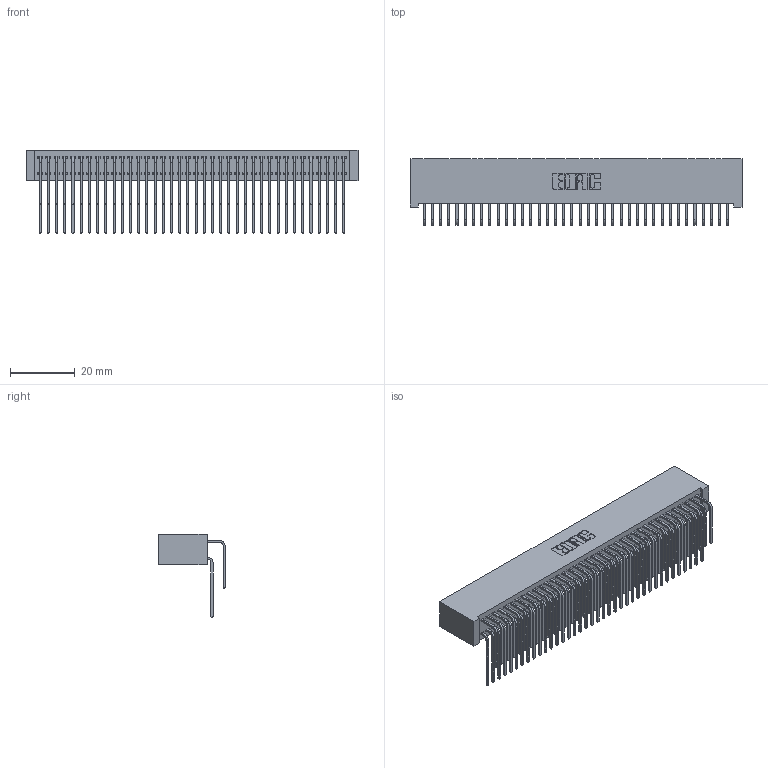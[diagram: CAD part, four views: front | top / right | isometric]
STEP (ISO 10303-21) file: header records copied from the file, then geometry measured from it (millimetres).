
FILE_DESCRIPTION (( 'STEP AP203' ), '1' );
FILE_NAME ('392-076-559-201.STEP', '2018-08-18T01:47:36', ( '' ), ( '' ), 'SwSTEP 2.0', 'SolidWorks 2016', '' );
FILE_SCHEMA (( 'CONFIG_CONTROL_DESIGN' ));
Length unit declared in the file: inch
Products named in the file (4): 342 Part_Lugless; 345-292-001_558 559 Tail - 1; 345-292-001_559 Tail - 2; 392-076-559-201
Assembly tree (77 placements, depth 2):
  392-076-559-201
    342 Part_Lugless
    345-292-001_558 559 Tail - 1  x38
    345-292-001_559 Tail - 2  x38
Bounding box: 102.77 x 20.64 x 25.78 mm (x, y, z)
Volume: 10092.7 mm3; surface area: 18759.4 mm2
Topology: 77 solids, 77 shells, 4206 faces, 12511 edges, 8238 vertices
Faces by surface type: plane 2950, cylinder 1256
Entity records: 26339 total; most frequent: CARTESIAN_POINT 4417, ORIENTED_EDGE 4302, DIRECTION 3755, EDGE_CURVE 2151, VECTOR 1991, LINE 1991, VERTEX_POINT 1430, AXIS2_PLACEMENT_3D 882
